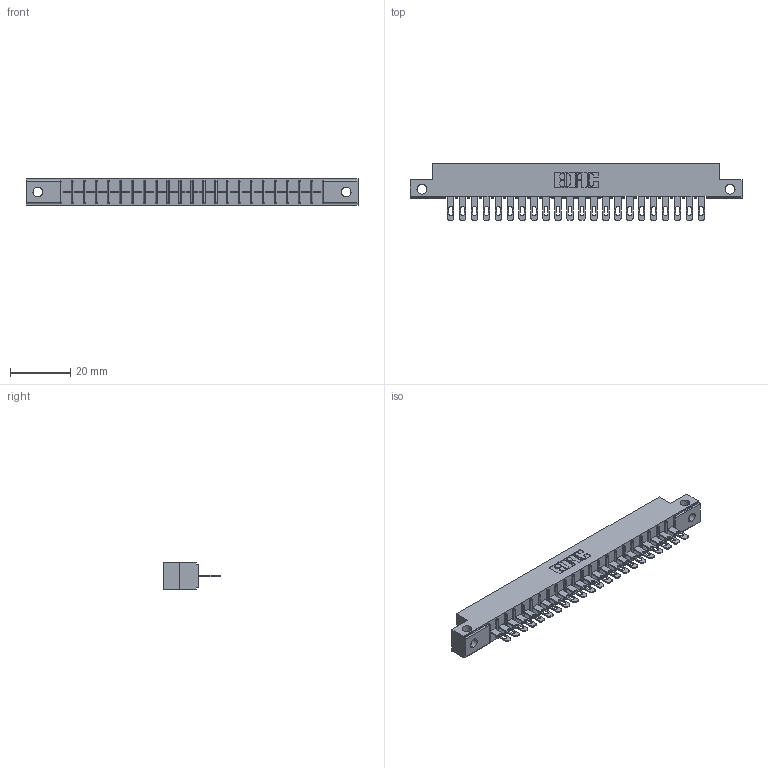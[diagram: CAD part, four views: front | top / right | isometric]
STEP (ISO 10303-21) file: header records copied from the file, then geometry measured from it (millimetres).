
FILE_DESCRIPTION (( 'STEP AP203' ), '1' );
FILE_NAME ('356-022-500-112.STEP', '2020-09-20T22:21:40', ( '' ), ( '' ), 'SwSTEP 2.0', 'SolidWorks 2020', '' );
FILE_SCHEMA (( 'CONFIG_CONTROL_DESIGN' ));
Length unit declared in the file: inch
Products named in the file (3): 356-022-500-112; 306-290-001_100; 306 Part_.128 Dia
Assembly tree (23 placements, depth 2):
  356-022-500-112
    306 Part_.128 Dia
    306-290-001_100  x22
Bounding box: 110.19 x 18.87 x 8.71 mm (x, y, z)
Volume: 7467.1 mm3; surface area: 11344.4 mm2
Topology: 23 solids, 23 shells, 1800 faces, 5082 edges, 3264 vertices
Faces by surface type: plane 1168, cylinder 544, sphere 88
Entity records: 23677 total; most frequent: CARTESIAN_POINT 4021, ORIENTED_EDGE 3940, DIRECTION 3906, EDGE_CURVE 1970, LINE 1512, VECTOR 1512, VERTEX_POINT 1248, AXIS2_PLACEMENT_3D 1197
